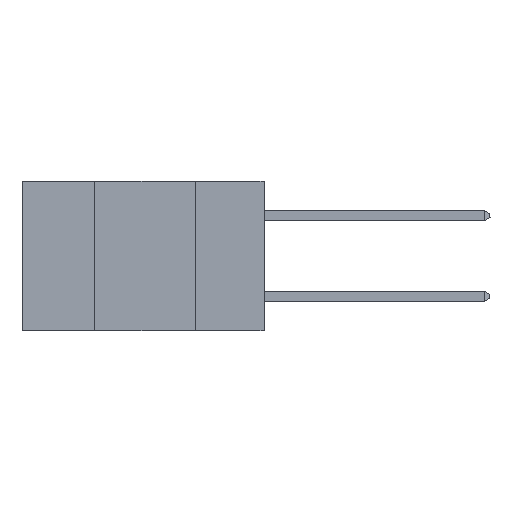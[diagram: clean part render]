
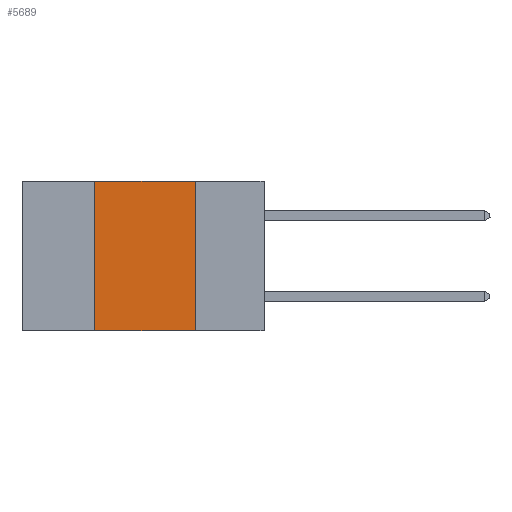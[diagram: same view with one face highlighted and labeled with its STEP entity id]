
A CAD part, left-side view. The second image highlights one B-rep face of the part: STEP entity #5689.
In plain terms, the highlighted planar face has unit normal (-1, 0, 0).
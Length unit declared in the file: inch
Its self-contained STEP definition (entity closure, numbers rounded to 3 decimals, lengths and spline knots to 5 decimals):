
#465 = CARTESIAN_POINT ( 'NONE',  ( 0., 0.6, 0. ) ) ;
#690 = EDGE_CURVE ( 'NONE', #3528, #3149, #14692, .T. ) ;
#1194 = VECTOR ( 'NONE', #4150, 39.37008 ) ;
#1637 = CARTESIAN_POINT ( 'NONE',  ( 0., 0.42, 0. ) ) ;
#1867 = VECTOR ( 'NONE', #3366, 39.37008 ) ;
#1874 = CARTESIAN_POINT ( 'NONE',  ( 0., 0.17, 0. ) ) ;
#1921 = EDGE_CURVE ( 'NONE', #14724, #3528, #13206, .T. ) ;
#2174 = AXIS2_PLACEMENT_3D ( 'NONE', #5647, #5544, #12586 ) ;
#3007 = ORIENTED_EDGE ( 'NONE', *, *, #5638, .F. ) ;
#3149 = VERTEX_POINT ( 'NONE', #13966 ) ;
#3328 = EDGE_CURVE ( 'NONE', #14724, #6946, #8294, .T. ) ;
#3366 = DIRECTION ( 'NONE',  ( 0., -1., 0. ) ) ;
#3528 = VERTEX_POINT ( 'NONE', #4451 ) ;
#3631 = ORIENTED_EDGE ( 'NONE', *, *, #3328, .T. ) ;
#4150 = DIRECTION ( 'NONE',  ( 0., 0., -1. ) ) ;
#4435 = ORIENTED_EDGE ( 'NONE', *, *, #690, .F. ) ;
#4439 = PLANE ( 'NONE',  #2174 ) ;
#4451 = CARTESIAN_POINT ( 'NONE',  ( 0., 0.42, 0. ) ) ;
#4737 = VECTOR ( 'NONE', #13522, 39.37008 ) ;
#5269 = LINE ( 'NONE', #1874, #1194 ) ;
#5544 = DIRECTION ( 'NONE',  ( 1., 0., 0. ) ) ;
#5638 = EDGE_CURVE ( 'NONE', #3149, #6946, #5269, .T. ) ;
#5647 = CARTESIAN_POINT ( 'NONE',  ( 0., 0.6, 0. ) ) ;
#5689 = ADVANCED_FACE ( 'NONE', ( #9455 ), #4439, .F. ) ;
#6006 = CARTESIAN_POINT ( 'NONE',  ( 0., 0.17, -0.37 ) ) ;
#6357 = VECTOR ( 'NONE', #14316, 39.37008 ) ;
#6946 = VERTEX_POINT ( 'NONE', #6006 ) ;
#8294 = LINE ( 'NONE', #13952, #1867 ) ;
#9455 = FACE_OUTER_BOUND ( 'NONE', #14561, .T. ) ;
#11965 = CARTESIAN_POINT ( 'NONE',  ( 0., 0.42, -0.37 ) ) ;
#12586 = DIRECTION ( 'NONE',  ( 0., 0., -1. ) ) ;
#13206 = LINE ( 'NONE', #1637, #6357 ) ;
#13522 = DIRECTION ( 'NONE',  ( 0., -1., 0. ) ) ;
#13952 = CARTESIAN_POINT ( 'NONE',  ( 0., 0.6, -0.37 ) ) ;
#13966 = CARTESIAN_POINT ( 'NONE',  ( 0., 0.17, 0. ) ) ;
#14145 = ORIENTED_EDGE ( 'NONE', *, *, #1921, .F. ) ;
#14316 = DIRECTION ( 'NONE',  ( 0., 0., 1. ) ) ;
#14561 = EDGE_LOOP ( 'NONE', ( #3007, #4435, #14145, #3631 ) ) ;
#14692 = LINE ( 'NONE', #465, #4737 ) ;
#14724 = VERTEX_POINT ( 'NONE', #11965 ) ;
